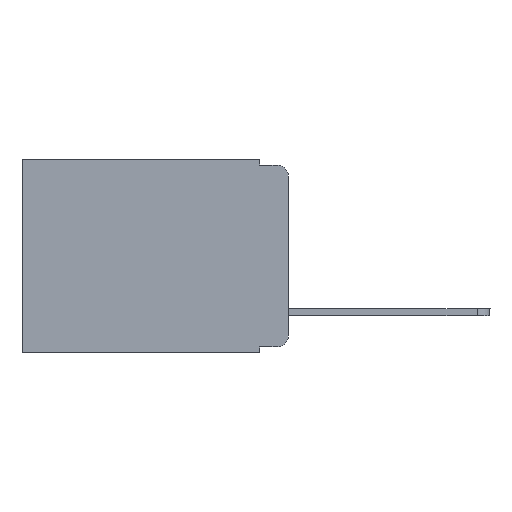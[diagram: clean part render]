
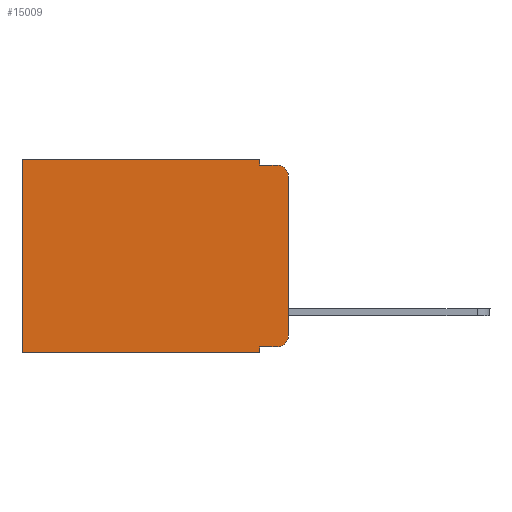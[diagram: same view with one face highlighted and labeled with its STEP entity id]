
A CAD part, left-side view. The second image highlights one B-rep face of the part: STEP entity #15009.
In plain terms, the highlighted planar face has unit normal (-1, 0, 0).
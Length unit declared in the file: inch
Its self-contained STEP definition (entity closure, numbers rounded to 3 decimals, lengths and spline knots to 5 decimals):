
#339 = DIRECTION ( 'NONE',  ( 0., -1., 0. ) ) ;
#544 = EDGE_CURVE ( 'NONE', #9276, #4862, #8451, .T. ) ;
#572 = VECTOR ( 'NONE', #15429, 39.37008 ) ;
#1098 = VECTOR ( 'NONE', #9968, 39.37008 ) ;
#1343 = LINE ( 'NONE', #5211, #8208 ) ;
#1601 = DIRECTION ( 'NONE',  ( 0., 0., -1. ) ) ;
#1794 = LINE ( 'NONE', #15326, #572 ) ;
#2127 = CARTESIAN_POINT ( 'NONE',  ( 0.298, 0.02, -0.313 ) ) ;
#2267 = VERTEX_POINT ( 'NONE', #7192 ) ;
#2491 = EDGE_CURVE ( 'NONE', #11501, #9276, #4767, .T. ) ;
#2542 = EDGE_CURVE ( 'NONE', #2267, #4862, #7397, .T. ) ;
#2783 = AXIS2_PLACEMENT_3D ( 'NONE', #2127, #3501, #7307 ) ;
#3026 = EDGE_CURVE ( 'NONE', #3625, #14522, #10735, .T. ) ;
#3142 = CARTESIAN_POINT ( 'NONE',  ( 0.298, 0.473, -0.343 ) ) ;
#3254 = DIRECTION ( 'NONE',  ( 0., 1., 0. ) ) ;
#3501 = DIRECTION ( 'NONE',  ( -1., 0., 0. ) ) ;
#3625 = VERTEX_POINT ( 'NONE', #14683 ) ;
#3823 = VECTOR ( 'NONE', #3254, 39.37008 ) ;
#4057 = VERTEX_POINT ( 'NONE', #9289 ) ;
#4116 = PLANE ( 'NONE',  #8888 ) ;
#4437 = ORIENTED_EDGE ( 'NONE', *, *, #2542, .T. ) ;
#4438 = LINE ( 'NONE', #14806, #10250 ) ;
#4505 = EDGE_CURVE ( 'NONE', #4057, #8508, #13323, .T. ) ;
#4655 = DIRECTION ( 'NONE',  ( 0., 1., 0. ) ) ;
#4767 = LINE ( 'NONE', #4776, #1098 ) ;
#4776 = CARTESIAN_POINT ( 'NONE',  ( 0.298, 0.051, 0. ) ) ;
#4862 = VERTEX_POINT ( 'NONE', #3142 ) ;
#5211 = CARTESIAN_POINT ( 'NONE',  ( 0.298, 0., 0. ) ) ;
#5339 = CARTESIAN_POINT ( 'NONE',  ( 0.298, 0.051, 0. ) ) ;
#5960 = CARTESIAN_POINT ( 'NONE',  ( 0.298, 0.473, 0. ) ) ;
#6384 = VERTEX_POINT ( 'NONE', #5339 ) ;
#6457 = CARTESIAN_POINT ( 'NONE',  ( 0.298, 0., -0.03 ) ) ;
#6513 = DIRECTION ( 'NONE',  ( 0., 0., -1. ) ) ;
#6798 = CARTESIAN_POINT ( 'NONE',  ( 0.298, 0., 0. ) ) ;
#6843 = DIRECTION ( 'NONE',  ( 1., 0., 0. ) ) ;
#6859 = ORIENTED_EDGE ( 'NONE', *, *, #2491, .F. ) ;
#6876 = CIRCLE ( 'NONE', #7231, 0.02 ) ;
#6977 = VERTEX_POINT ( 'NONE', #6457 ) ;
#7122 = ORIENTED_EDGE ( 'NONE', *, *, #4505, .F. ) ;
#7192 = CARTESIAN_POINT ( 'NONE',  ( 0.298, 0.473, 0. ) ) ;
#7231 = AXIS2_PLACEMENT_3D ( 'NONE', #11171, #9936, #11111 ) ;
#7307 = DIRECTION ( 'NONE',  ( 0., 0., -1. ) ) ;
#7397 = LINE ( 'NONE', #5960, #13768 ) ;
#7445 = CARTESIAN_POINT ( 'NONE',  ( 0.298, 0.051, -0.343 ) ) ;
#8089 = CARTESIAN_POINT ( 'NONE',  ( 0.298, 0.051, -0.01 ) ) ;
#8208 = VECTOR ( 'NONE', #6513, 39.37008 ) ;
#8289 = CARTESIAN_POINT ( 'NONE',  ( 0.298, 0., -0.313 ) ) ;
#8292 = CARTESIAN_POINT ( 'NONE',  ( 0.298, 0.02, -0.01 ) ) ;
#8451 = LINE ( 'NONE', #16291, #3823 ) ;
#8466 = VECTOR ( 'NONE', #12504, 39.37008 ) ;
#8508 = VERTEX_POINT ( 'NONE', #8292 ) ;
#8888 = AXIS2_PLACEMENT_3D ( 'NONE', #6798, #6843, #1601 ) ;
#9276 = VERTEX_POINT ( 'NONE', #7445 ) ;
#9289 = CARTESIAN_POINT ( 'NONE',  ( 0.298, 0.051, -0.01 ) ) ;
#9838 = ORIENTED_EDGE ( 'NONE', *, *, #3026, .T. ) ;
#9912 = VECTOR ( 'NONE', #339, 39.37008 ) ;
#9936 = DIRECTION ( 'NONE',  ( -1., 0., 0. ) ) ;
#9968 = DIRECTION ( 'NONE',  ( 0., 0., -1. ) ) ;
#10105 = EDGE_CURVE ( 'NONE', #6384, #4057, #1794, .T. ) ;
#10250 = VECTOR ( 'NONE', #4655, 39.37008 ) ;
#10735 = CIRCLE ( 'NONE', #2783, 0.02 ) ;
#11111 = DIRECTION ( 'NONE',  ( 0., 0., -1. ) ) ;
#11171 = CARTESIAN_POINT ( 'NONE',  ( 0.298, 0.02, -0.03 ) ) ;
#11458 = EDGE_CURVE ( 'NONE', #6977, #8508, #6876, .T. ) ;
#11501 = VERTEX_POINT ( 'NONE', #13689 ) ;
#12057 = ORIENTED_EDGE ( 'NONE', *, *, #11458, .T. ) ;
#12253 = ORIENTED_EDGE ( 'NONE', *, *, #544, .F. ) ;
#12504 = DIRECTION ( 'NONE',  ( 0., -1., 0. ) ) ;
#13178 = FACE_OUTER_BOUND ( 'NONE', #13679, .T. ) ;
#13189 = EDGE_CURVE ( 'NONE', #11501, #3625, #15630, .T. ) ;
#13285 = EDGE_CURVE ( 'NONE', #6384, #2267, #4438, .T. ) ;
#13323 = LINE ( 'NONE', #8089, #9912 ) ;
#13611 = CARTESIAN_POINT ( 'NONE',  ( 0.298, 0.051, -0.333 ) ) ;
#13679 = EDGE_LOOP ( 'NONE', ( #13978, #12057, #7122, #14733, #15160, #4437, #12253, #6859, #14562, #9838 ) ) ;
#13689 = CARTESIAN_POINT ( 'NONE',  ( 0.298, 0.051, -0.333 ) ) ;
#13768 = VECTOR ( 'NONE', #14860, 39.37008 ) ;
#13978 = ORIENTED_EDGE ( 'NONE', *, *, #14897, .F. ) ;
#14522 = VERTEX_POINT ( 'NONE', #8289 ) ;
#14562 = ORIENTED_EDGE ( 'NONE', *, *, #13189, .T. ) ;
#14683 = CARTESIAN_POINT ( 'NONE',  ( 0.298, 0.02, -0.333 ) ) ;
#14733 = ORIENTED_EDGE ( 'NONE', *, *, #10105, .F. ) ;
#14806 = CARTESIAN_POINT ( 'NONE',  ( 0.298, 0., 0. ) ) ;
#14860 = DIRECTION ( 'NONE',  ( 0., 0., -1. ) ) ;
#14897 = EDGE_CURVE ( 'NONE', #6977, #14522, #1343, .T. ) ;
#15009 = ADVANCED_FACE ( 'NONE', ( #13178 ), #4116, .F. ) ;
#15160 = ORIENTED_EDGE ( 'NONE', *, *, #13285, .T. ) ;
#15326 = CARTESIAN_POINT ( 'NONE',  ( 0.298, 0.051, 0. ) ) ;
#15429 = DIRECTION ( 'NONE',  ( 0., 0., -1. ) ) ;
#15630 = LINE ( 'NONE', #13611, #8466 ) ;
#16291 = CARTESIAN_POINT ( 'NONE',  ( 0.298, 0., -0.343 ) ) ;
